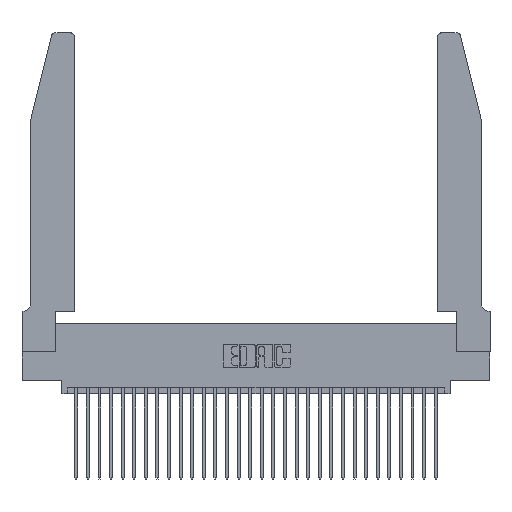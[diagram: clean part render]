
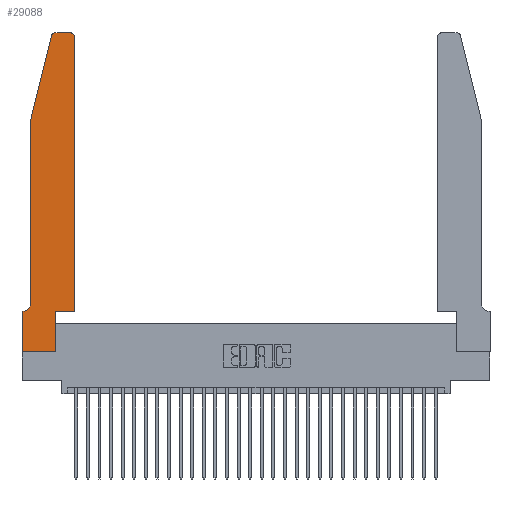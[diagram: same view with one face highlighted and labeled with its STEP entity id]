
A CAD part, top view. The second image highlights one B-rep face of the part: STEP entity #29088.
In plain terms, the highlighted planar face has unit normal (0, 0, 1).
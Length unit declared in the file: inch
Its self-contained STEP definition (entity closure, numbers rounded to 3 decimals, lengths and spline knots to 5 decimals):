
#78 = ORIENTED_EDGE ( 'NONE', *, *, #23026, .T. ) ;
#1340 = DIRECTION ( 'NONE',  ( -1., 0., 0. ) ) ;
#1448 = LINE ( 'NONE', #14271, #20324 ) ;
#1471 = LINE ( 'NONE', #23869, #23033 ) ;
#2178 = DIRECTION ( 'NONE',  ( 0., -1., 0. ) ) ;
#2429 = DIRECTION ( 'NONE',  ( 1., 0., 0. ) ) ;
#2499 = FACE_OUTER_BOUND ( 'NONE', #11313, .T. ) ;
#2973 = EDGE_CURVE ( 'NONE', #17078, #25780, #14932, .T. ) ;
#3313 = VECTOR ( 'NONE', #11819, 39.37008 ) ;
#3642 = ORIENTED_EDGE ( 'NONE', *, *, #6524, .T. ) ;
#3657 = CARTESIAN_POINT ( 'NONE',  ( 0.284, 2.75, 0.37 ) ) ;
#4189 = ORIENTED_EDGE ( 'NONE', *, *, #21435, .T. ) ;
#4409 = CIRCLE ( 'NONE', #28309, 0.03 ) ;
#5205 = DIRECTION ( 'NONE',  ( 1., 0., 0. ) ) ;
#5549 = DIRECTION ( 'NONE',  ( 0., -1., 0. ) ) ;
#5752 = CARTESIAN_POINT ( 'NONE',  ( 0.4205, 2.75, 0.37 ) ) ;
#5846 = DIRECTION ( 'NONE',  ( 0., 0., 1. ) ) ;
#6283 = CIRCLE ( 'NONE', #17580, 0.03 ) ;
#6448 = ORIENTED_EDGE ( 'NONE', *, *, #13194, .T. ) ;
#6513 = CARTESIAN_POINT ( 'NONE',  ( 0.4505, 0.35, 0.37 ) ) ;
#6524 = EDGE_CURVE ( 'NONE', #26636, #24566, #1471, .T. ) ;
#6703 = CARTESIAN_POINT ( 'NONE',  ( 0.0755, 2., 0.37 ) ) ;
#6991 = AXIS2_PLACEMENT_3D ( 'NONE', #22465, #19941, #5205 ) ;
#8013 = VECTOR ( 'NONE', #8956, 39.37008 ) ;
#8475 = LINE ( 'NONE', #9338, #30512 ) ;
#8490 = CARTESIAN_POINT ( 'NONE',  ( 0.4205, 2.72, 0.37 ) ) ;
#8660 = CARTESIAN_POINT ( 'NONE',  ( 0.0055, 0.42, 0.37 ) ) ;
#8702 = CARTESIAN_POINT ( 'NONE',  ( 0.2865, 0.35, 0.37 ) ) ;
#8956 = DIRECTION ( 'NONE',  ( 0., 1., 0. ) ) ;
#9338 = CARTESIAN_POINT ( 'NONE',  ( 0.0755, 2., 0.37 ) ) ;
#10333 = ORIENTED_EDGE ( 'NONE', *, *, #19389, .T. ) ;
#10419 = CARTESIAN_POINT ( 'NONE',  ( 0.4505, 0.35, 0.37 ) ) ;
#11313 = EDGE_LOOP ( 'NONE', ( #78, #17673, #15167, #16351, #22835, #14351, #17643, #6448, #3642, #4189, #10333, #29724 ) ) ;
#11819 = DIRECTION ( 'NONE',  ( 1., 0., 0. ) ) ;
#12041 = CARTESIAN_POINT ( 'NONE',  ( 0.25487, 2.72718, 0.37 ) ) ;
#12234 = DIRECTION ( 'NONE',  ( 0., 0., 1. ) ) ;
#12407 = CARTESIAN_POINT ( 'NONE',  ( 0.4505, 2.72, 0.37 ) ) ;
#12458 = VERTEX_POINT ( 'NONE', #5752 ) ;
#12985 = VERTEX_POINT ( 'NONE', #10419 ) ;
#13194 = EDGE_CURVE ( 'NONE', #25780, #26636, #30228, .T. ) ;
#13242 = EDGE_CURVE ( 'NONE', #26407, #17078, #1448, .T. ) ;
#13288 = CARTESIAN_POINT ( 'NONE',  ( 0., 0., 0.37 ) ) ;
#13503 = EDGE_CURVE ( 'NONE', #15018, #22672, #6283, .T. ) ;
#13798 = VECTOR ( 'NONE', #5549, 39.37008 ) ;
#13931 = DIRECTION ( 'NONE',  ( -1., 0., 0. ) ) ;
#14271 = CARTESIAN_POINT ( 'NONE',  ( 0.0755, 0.35, 0.37 ) ) ;
#14351 = ORIENTED_EDGE ( 'NONE', *, *, #13242, .T. ) ;
#14498 = LINE ( 'NONE', #6513, #8013 ) ;
#14932 = LINE ( 'NONE', #13288, #13798 ) ;
#15018 = VERTEX_POINT ( 'NONE', #3657 ) ;
#15066 = EDGE_CURVE ( 'NONE', #21242, #29618, #8475, .T. ) ;
#15167 = ORIENTED_EDGE ( 'NONE', *, *, #21966, .T. ) ;
#15834 = CARTESIAN_POINT ( 'NONE',  ( 0.0055, 0.35, 0.37 ) ) ;
#15838 = AXIS2_PLACEMENT_3D ( 'NONE', #8660, #20856, #17773 ) ;
#16351 = ORIENTED_EDGE ( 'NONE', *, *, #15066, .T. ) ;
#16435 = DIRECTION ( 'NONE',  ( 0., 1., 0. ) ) ;
#16773 = CARTESIAN_POINT ( 'NONE',  ( 0.4505, 0.35, 0.37 ) ) ;
#17078 = VERTEX_POINT ( 'NONE', #24770 ) ;
#17231 = EDGE_CURVE ( 'NONE', #29618, #26407, #21845, .T. ) ;
#17398 = VECTOR ( 'NONE', #28980, 39.37008 ) ;
#17580 = AXIS2_PLACEMENT_3D ( 'NONE', #19145, #12234, #2429 ) ;
#17643 = ORIENTED_EDGE ( 'NONE', *, *, #2973, .T. ) ;
#17673 = ORIENTED_EDGE ( 'NONE', *, *, #13503, .T. ) ;
#17773 = DIRECTION ( 'NONE',  ( -1., 0., 0. ) ) ;
#18128 = LINE ( 'NONE', #27985, #23837 ) ;
#19145 = CARTESIAN_POINT ( 'NONE',  ( 0.284, 2.72, 0.37 ) ) ;
#19227 = CARTESIAN_POINT ( 'NONE',  ( 0.2865, 0., 0.37 ) ) ;
#19389 = EDGE_CURVE ( 'NONE', #12985, #30248, #14498, .T. ) ;
#19734 = PLANE ( 'NONE',  #6991 ) ;
#19941 = DIRECTION ( 'NONE',  ( 0., 0., 1. ) ) ;
#20324 = VECTOR ( 'NONE', #1340, 39.37008 ) ;
#20768 = DIRECTION ( 'NONE',  ( -0.239, -0.971, 0. ) ) ;
#20856 = DIRECTION ( 'NONE',  ( 0., 0., -1. ) ) ;
#21242 = VERTEX_POINT ( 'NONE', #6703 ) ;
#21435 = EDGE_CURVE ( 'NONE', #24566, #12985, #24603, .T. ) ;
#21845 = CIRCLE ( 'NONE', #15838, 0.07 ) ;
#21966 = EDGE_CURVE ( 'NONE', #22672, #21242, #18128, .T. ) ;
#22465 = CARTESIAN_POINT ( 'NONE',  ( 0., 0.35, 0.37 ) ) ;
#22672 = VERTEX_POINT ( 'NONE', #12041 ) ;
#22685 = DIRECTION ( 'NONE',  ( 1., 0., 0. ) ) ;
#22835 = ORIENTED_EDGE ( 'NONE', *, *, #17231, .T. ) ;
#23026 = EDGE_CURVE ( 'NONE', #12458, #15018, #29706, .T. ) ;
#23033 = VECTOR ( 'NONE', #16435, 39.37008 ) ;
#23261 = CARTESIAN_POINT ( 'NONE',  ( 0.2605, 2.75, 0.37 ) ) ;
#23837 = VECTOR ( 'NONE', #20768, 39.37008 ) ;
#23869 = CARTESIAN_POINT ( 'NONE',  ( 0.2865, 0.35, 0.37 ) ) ;
#23966 = CARTESIAN_POINT ( 'NONE',  ( 0.0755, 0.42, 0.37 ) ) ;
#24566 = VERTEX_POINT ( 'NONE', #8702 ) ;
#24603 = LINE ( 'NONE', #16773, #17398 ) ;
#24770 = CARTESIAN_POINT ( 'NONE',  ( 0., 0.35, 0.37 ) ) ;
#25525 = VECTOR ( 'NONE', #13931, 39.37008 ) ;
#25780 = VERTEX_POINT ( 'NONE', #25929 ) ;
#25929 = CARTESIAN_POINT ( 'NONE',  ( 0., 0., 0.37 ) ) ;
#26407 = VERTEX_POINT ( 'NONE', #15834 ) ;
#26545 = CARTESIAN_POINT ( 'NONE',  ( 0., 0., 0.37 ) ) ;
#26636 = VERTEX_POINT ( 'NONE', #19227 ) ;
#27255 = EDGE_CURVE ( 'NONE', #30248, #12458, #4409, .T. ) ;
#27985 = CARTESIAN_POINT ( 'NONE',  ( 0.0755, 2., 0.37 ) ) ;
#28309 = AXIS2_PLACEMENT_3D ( 'NONE', #8490, #5846, #22685 ) ;
#28980 = DIRECTION ( 'NONE',  ( 1., 0., 0. ) ) ;
#29088 = ADVANCED_FACE ( 'NONE', ( #2499 ), #19734, .T. ) ;
#29618 = VERTEX_POINT ( 'NONE', #23966 ) ;
#29706 = LINE ( 'NONE', #23261, #25525 ) ;
#29724 = ORIENTED_EDGE ( 'NONE', *, *, #27255, .T. ) ;
#30228 = LINE ( 'NONE', #26545, #3313 ) ;
#30248 = VERTEX_POINT ( 'NONE', #12407 ) ;
#30512 = VECTOR ( 'NONE', #2178, 39.37008 ) ;
